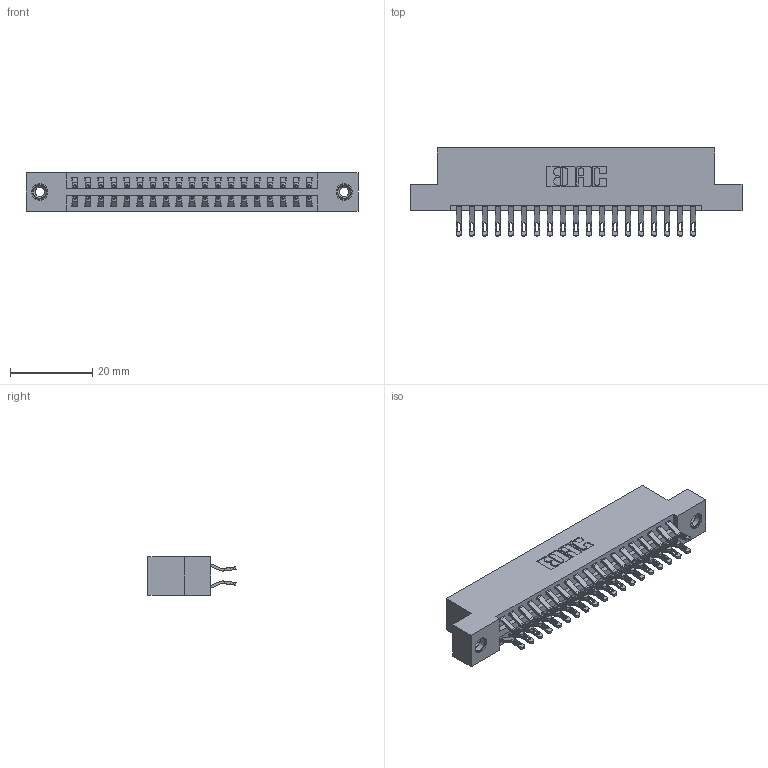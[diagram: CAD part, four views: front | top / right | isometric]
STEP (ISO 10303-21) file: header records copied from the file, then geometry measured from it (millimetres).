
FILE_DESCRIPTION (( 'STEP AP203' ), '1' );
FILE_NAME ('396-038-555-208.STEP', '2018-09-06T08:45:18', ( '' ), ( '' ), 'SwSTEP 2.0', 'SolidWorks 2016', '' );
FILE_SCHEMA (( 'CONFIG_CONTROL_DESIGN' ));
Length unit declared in the file: inch
Products named in the file (4): 346 Part_Flush Mounting Lugs - 0.156 Dia-TI; 345-292-001_555 Tail; 345-250-001_345-250-003-102; 396-038-555-208
Assembly tree (41 placements, depth 2):
  396-038-555-208
    346 Part_Flush Mounting Lugs - 0.156 Dia-TI
    345-292-001_555 Tail  x38
    345-250-001_345-250-003-102  x2
Bounding box: 80.9 x 21.46 x 9.4 mm (x, y, z)
Volume: 7813.7 mm3; surface area: 10791.9 mm2
Topology: 41 solids, 41 shells, 2386 faces, 7419 edges, 4938 vertices
Faces by surface type: plane 1362, cylinder 1008, cone 12, torus 4
Entity records: 17008 total; most frequent: CARTESIAN_POINT 2853, ORIENTED_EDGE 2750, DIRECTION 2561, EDGE_CURVE 1375, VECTOR 1127, LINE 1127, VERTEX_POINT 912, AXIS2_PLACEMENT_3D 717
